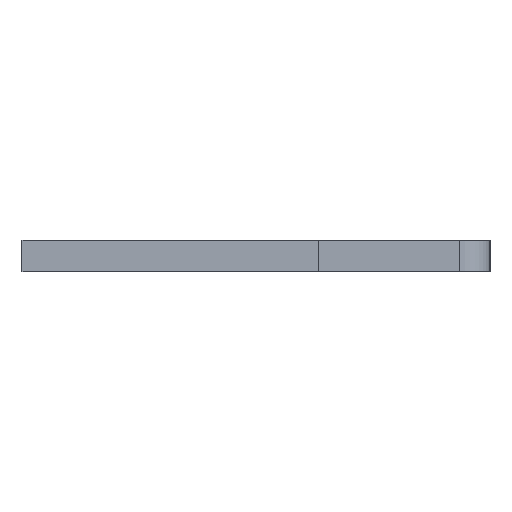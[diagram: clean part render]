
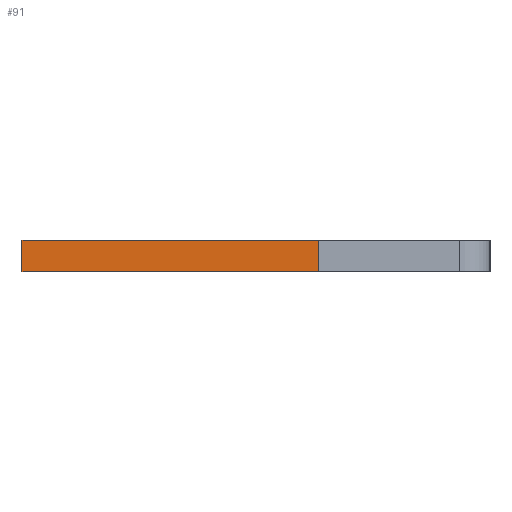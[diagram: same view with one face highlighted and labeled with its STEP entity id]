
A CAD part, left-side view. The second image highlights one B-rep face of the part: STEP entity #91.
In plain terms, the highlighted face is planar.
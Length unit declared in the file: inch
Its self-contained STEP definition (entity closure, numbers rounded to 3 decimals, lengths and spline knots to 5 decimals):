
#47 = EDGE_CURVE ( 'NONE', #1468, #247, #1643, .T. ) ;
#91 = ADVANCED_FACE ( 'NONE', ( #1763 ), #211, .F. ) ;
#172 = VECTOR ( 'NONE', #701, 39.37008 ) ;
#211 = PLANE ( 'NONE',  #567 ) ;
#247 = VERTEX_POINT ( 'NONE', #1410 ) ;
#254 = DIRECTION ( 'NONE',  ( 0., 1., 0. ) ) ;
#293 = EDGE_CURVE ( 'NONE', #1159, #1328, #1186, .T. ) ;
#344 = DIRECTION ( 'NONE',  ( 1., 0., 0. ) ) ;
#373 = CARTESIAN_POINT ( 'NONE',  ( 0.01, -0.04, -0.04 ) ) ;
#471 = CARTESIAN_POINT ( 'NONE',  ( 0.01, -0.04, -0.04 ) ) ;
#497 = EDGE_LOOP ( 'NONE', ( #1700, #1107, #632, #675 ) ) ;
#544 = CARTESIAN_POINT ( 'NONE',  ( 0.01, 0.15, -0.04 ) ) ;
#567 = AXIS2_PLACEMENT_3D ( 'NONE', #780, #1215, #344 ) ;
#632 = ORIENTED_EDGE ( 'NONE', *, *, #293, .F. ) ;
#640 = VECTOR ( 'NONE', #1086, 39.37008 ) ;
#675 = ORIENTED_EDGE ( 'NONE', *, *, #1843, .T. ) ;
#701 = DIRECTION ( 'NONE',  ( -1., 0., 0. ) ) ;
#705 = VECTOR ( 'NONE', #786, 39.37008 ) ;
#780 = CARTESIAN_POINT ( 'NONE',  ( 0.01, 0.15, -0.04 ) ) ;
#786 = DIRECTION ( 'NONE',  ( 0., 1., 0. ) ) ;
#796 = VECTOR ( 'NONE', #254, 39.37008 ) ;
#870 = LINE ( 'NONE', #1711, #640 ) ;
#1086 = DIRECTION ( 'NONE',  ( -1., 0., 0. ) ) ;
#1093 = CARTESIAN_POINT ( 'NONE',  ( -0.01, 0.15, -0.04 ) ) ;
#1107 = ORIENTED_EDGE ( 'NONE', *, *, #1710, .F. ) ;
#1159 = VERTEX_POINT ( 'NONE', #471 ) ;
#1186 = LINE ( 'NONE', #544, #796 ) ;
#1215 = DIRECTION ( 'NONE',  ( 0., 0., 1. ) ) ;
#1328 = VERTEX_POINT ( 'NONE', #1816 ) ;
#1410 = CARTESIAN_POINT ( 'NONE',  ( -0.01, 0.15, -0.04 ) ) ;
#1468 = VERTEX_POINT ( 'NONE', #1702 ) ;
#1643 = LINE ( 'NONE', #1093, #705 ) ;
#1700 = ORIENTED_EDGE ( 'NONE', *, *, #47, .T. ) ;
#1702 = CARTESIAN_POINT ( 'NONE',  ( -0.01, -0.04, -0.04 ) ) ;
#1710 = EDGE_CURVE ( 'NONE', #1328, #247, #870, .T. ) ;
#1711 = CARTESIAN_POINT ( 'NONE',  ( 0.01, 0.15, -0.04 ) ) ;
#1763 = FACE_OUTER_BOUND ( 'NONE', #497, .T. ) ;
#1816 = CARTESIAN_POINT ( 'NONE',  ( 0.01, 0.15, -0.04 ) ) ;
#1836 = LINE ( 'NONE', #373, #172 ) ;
#1843 = EDGE_CURVE ( 'NONE', #1159, #1468, #1836, .T. ) ;
